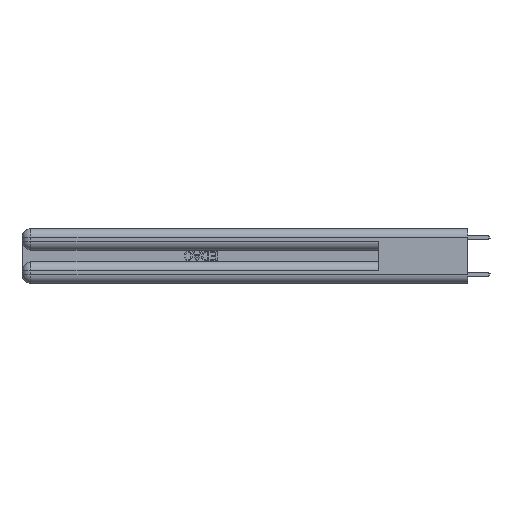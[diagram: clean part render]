
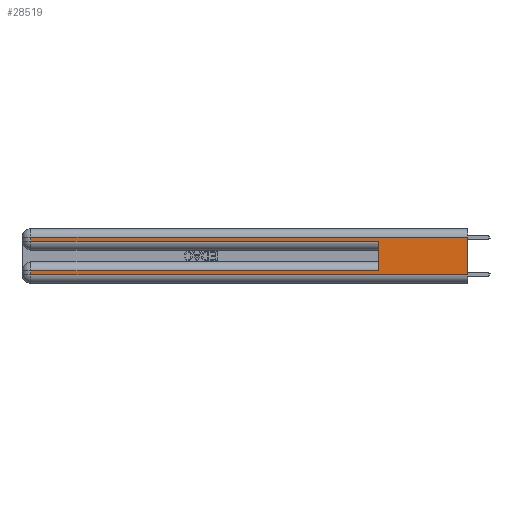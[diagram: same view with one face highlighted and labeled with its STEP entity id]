
A CAD part, left-side view. The second image highlights one B-rep face of the part: STEP entity #28519.
In plain terms, the highlighted planar face has unit normal (-1, 0, 0).
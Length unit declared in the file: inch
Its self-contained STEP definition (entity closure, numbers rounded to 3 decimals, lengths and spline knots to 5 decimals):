
#985 = PLANE ( 'NONE',  #31073 ) ;
#1600 = VERTEX_POINT ( 'NONE', #30134 ) ;
#2096 = DIRECTION ( 'NONE',  ( 0., 1., 0. ) ) ;
#2158 = CARTESIAN_POINT ( 'NONE',  ( 0., 0., 0.285 ) ) ;
#2822 = EDGE_CURVE ( 'NONE', #14843, #9148, #5550, .T. ) ;
#4123 = ORIENTED_EDGE ( 'NONE', *, *, #30241, .T. ) ;
#4706 = DIRECTION ( 'NONE',  ( 0., -1., 0. ) ) ;
#5116 = VERTEX_POINT ( 'NONE', #27692 ) ;
#5144 = LINE ( 'NONE', #27756, #19471 ) ;
#5550 = LINE ( 'NONE', #15892, #21054 ) ;
#6930 = LINE ( 'NONE', #2158, #21678 ) ;
#8433 = CARTESIAN_POINT ( 'NONE',  ( 0., 0.6, 0.285 ) ) ;
#8682 = CARTESIAN_POINT ( 'NONE',  ( 0., 0.6, 0.145 ) ) ;
#9148 = VERTEX_POINT ( 'NONE', #28441 ) ;
#9391 = EDGE_CURVE ( 'NONE', #32163, #32078, #24845, .T. ) ;
#9956 = LINE ( 'NONE', #25429, #10326 ) ;
#10326 = VECTOR ( 'NONE', #12518, 39.37008 ) ;
#10636 = DIRECTION ( 'NONE',  ( 0., 0., -1. ) ) ;
#11854 = CARTESIAN_POINT ( 'NONE',  ( 0., 0.6, 0.085 ) ) ;
#12463 = VECTOR ( 'NONE', #13441, 39.37008 ) ;
#12518 = DIRECTION ( 'NONE',  ( 0., 1., 0. ) ) ;
#13071 = VERTEX_POINT ( 'NONE', #8433 ) ;
#13441 = DIRECTION ( 'NONE',  ( 0., 0., 1. ) ) ;
#13908 = CARTESIAN_POINT ( 'NONE',  ( 0., 0., 0.37 ) ) ;
#14843 = VERTEX_POINT ( 'NONE', #23676 ) ;
#15892 = CARTESIAN_POINT ( 'NONE',  ( 0., 2.94, 0.37 ) ) ;
#16167 = ORIENTED_EDGE ( 'NONE', *, *, #24511, .T. ) ;
#17865 = VECTOR ( 'NONE', #18595, 39.37008 ) ;
#18392 = VERTEX_POINT ( 'NONE', #11854 ) ;
#18578 = EDGE_CURVE ( 'NONE', #1600, #13071, #6930, .T. ) ;
#18580 = ORIENTED_EDGE ( 'NONE', *, *, #9391, .F. ) ;
#18595 = DIRECTION ( 'NONE',  ( 0., -1., 0. ) ) ;
#18697 = EDGE_CURVE ( 'NONE', #9148, #32078, #28985, .T. ) ;
#19028 = LINE ( 'NONE', #8682, #12463 ) ;
#19127 = DIRECTION ( 'NONE',  ( 0., 0., -1. ) ) ;
#19130 = EDGE_CURVE ( 'NONE', #18392, #13071, #19028, .T. ) ;
#19295 = LINE ( 'NONE', #24053, #24604 ) ;
#19328 = FACE_OUTER_BOUND ( 'NONE', #23077, .T. ) ;
#19471 = VECTOR ( 'NONE', #2096, 39.37008 ) ;
#21054 = VECTOR ( 'NONE', #10636, 39.37008 ) ;
#21156 = CARTESIAN_POINT ( 'NONE',  ( 0., 0., 0.06 ) ) ;
#21357 = CARTESIAN_POINT ( 'NONE',  ( 0., 0., 0.06 ) ) ;
#21678 = VECTOR ( 'NONE', #4706, 39.37008 ) ;
#22136 = DIRECTION ( 'NONE',  ( 0., 0., -1. ) ) ;
#22379 = EDGE_CURVE ( 'NONE', #32163, #5116, #5144, .T. ) ;
#23077 = EDGE_LOOP ( 'NONE', ( #18580, #30200, #4123, #29656, #23554, #16167, #32026, #26544 ) ) ;
#23554 = ORIENTED_EDGE ( 'NONE', *, *, #19130, .F. ) ;
#23676 = CARTESIAN_POINT ( 'NONE',  ( 0., 2.94, 0.085 ) ) ;
#24053 = CARTESIAN_POINT ( 'NONE',  ( 0., 2.94, 0.37 ) ) ;
#24085 = DIRECTION ( 'NONE',  ( 0., 0., -1. ) ) ;
#24511 = EDGE_CURVE ( 'NONE', #18392, #14843, #9956, .T. ) ;
#24604 = VECTOR ( 'NONE', #19127, 39.37008 ) ;
#24845 = LINE ( 'NONE', #30308, #26208 ) ;
#24867 = CARTESIAN_POINT ( 'NONE',  ( 0., 0., 0.31 ) ) ;
#25429 = CARTESIAN_POINT ( 'NONE',  ( 0., 0., 0.085 ) ) ;
#26208 = VECTOR ( 'NONE', #22136, 39.37008 ) ;
#26544 = ORIENTED_EDGE ( 'NONE', *, *, #18697, .T. ) ;
#27692 = CARTESIAN_POINT ( 'NONE',  ( 0., 2.94, 0.31 ) ) ;
#27756 = CARTESIAN_POINT ( 'NONE',  ( 0., 0., 0.31 ) ) ;
#28441 = CARTESIAN_POINT ( 'NONE',  ( 0., 2.94, 0.06 ) ) ;
#28519 = ADVANCED_FACE ( 'NONE', ( #19328 ), #985, .F. ) ;
#28985 = LINE ( 'NONE', #21156, #17865 ) ;
#29549 = DIRECTION ( 'NONE',  ( 1., 0., 0. ) ) ;
#29656 = ORIENTED_EDGE ( 'NONE', *, *, #18578, .T. ) ;
#30134 = CARTESIAN_POINT ( 'NONE',  ( 0., 2.94, 0.285 ) ) ;
#30200 = ORIENTED_EDGE ( 'NONE', *, *, #22379, .T. ) ;
#30241 = EDGE_CURVE ( 'NONE', #5116, #1600, #19295, .T. ) ;
#30308 = CARTESIAN_POINT ( 'NONE',  ( 0., 0., 0.37 ) ) ;
#31073 = AXIS2_PLACEMENT_3D ( 'NONE', #13908, #29549, #24085 ) ;
#32026 = ORIENTED_EDGE ( 'NONE', *, *, #2822, .T. ) ;
#32078 = VERTEX_POINT ( 'NONE', #21357 ) ;
#32163 = VERTEX_POINT ( 'NONE', #24867 ) ;
